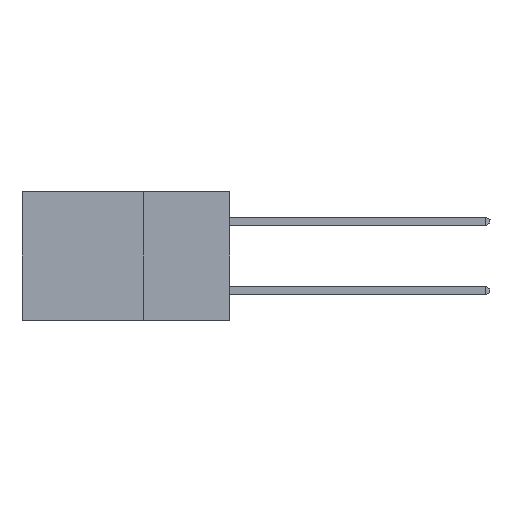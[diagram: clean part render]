
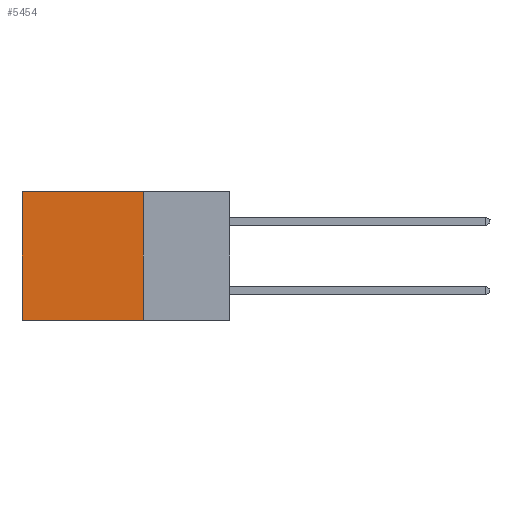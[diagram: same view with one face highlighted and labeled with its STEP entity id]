
A CAD part, left-side view. The second image highlights one B-rep face of the part: STEP entity #5454.
In plain terms, the highlighted planar face has unit normal (-1, 0, 0).
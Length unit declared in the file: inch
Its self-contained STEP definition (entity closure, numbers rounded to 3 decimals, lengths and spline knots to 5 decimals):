
#458 = CARTESIAN_POINT ( 'NONE',  ( 0.298, 0.25, 0. ) ) ;
#592 = PLANE ( 'NONE',  #22406 ) ;
#1752 = EDGE_CURVE ( 'NONE', #11318, #9129, #14719, .T. ) ;
#2717 = CARTESIAN_POINT ( 'NONE',  ( 0.298, 0.25, -0.37 ) ) ;
#3221 = CARTESIAN_POINT ( 'NONE',  ( 0.298, 0.6, -0.37 ) ) ;
#4415 = CARTESIAN_POINT ( 'NONE',  ( 0.298, 0.25, 0. ) ) ;
#4504 = EDGE_CURVE ( 'NONE', #11514, #21722, #30397, .T. ) ;
#4523 = DIRECTION ( 'NONE',  ( 0., 1., 0. ) ) ;
#5454 = ADVANCED_FACE ( 'NONE', ( #21950 ), #592, .F. ) ;
#5462 = LINE ( 'NONE', #11968, #6195 ) ;
#6195 = VECTOR ( 'NONE', #26225, 39.37008 ) ;
#7953 = CARTESIAN_POINT ( 'NONE',  ( 0.298, 0.6, 0. ) ) ;
#9041 = DIRECTION ( 'NONE',  ( 0., 0., -1. ) ) ;
#9129 = VERTEX_POINT ( 'NONE', #3221 ) ;
#10931 = VECTOR ( 'NONE', #4523, 39.37008 ) ;
#11121 = ORIENTED_EDGE ( 'NONE', *, *, #1752, .T. ) ;
#11318 = VERTEX_POINT ( 'NONE', #7953 ) ;
#11514 = VERTEX_POINT ( 'NONE', #4415 ) ;
#11968 = CARTESIAN_POINT ( 'NONE',  ( 0.298, 0.25, 0. ) ) ;
#13831 = VECTOR ( 'NONE', #21109, 39.37008 ) ;
#14478 = ORIENTED_EDGE ( 'NONE', *, *, #18356, .T. ) ;
#14674 = DIRECTION ( 'NONE',  ( 1., 0., 0. ) ) ;
#14719 = LINE ( 'NONE', #24206, #28016 ) ;
#15140 = EDGE_CURVE ( 'NONE', #21722, #9129, #16534, .T. ) ;
#16534 = LINE ( 'NONE', #18794, #10931 ) ;
#16572 = EDGE_LOOP ( 'NONE', ( #11121, #18132, #18493, #14478 ) ) ;
#18132 = ORIENTED_EDGE ( 'NONE', *, *, #15140, .F. ) ;
#18356 = EDGE_CURVE ( 'NONE', #11514, #11318, #5462, .T. ) ;
#18493 = ORIENTED_EDGE ( 'NONE', *, *, #4504, .F. ) ;
#18794 = CARTESIAN_POINT ( 'NONE',  ( 0.298, 0.25, -0.37 ) ) ;
#21109 = DIRECTION ( 'NONE',  ( 0., 0., -1. ) ) ;
#21709 = DIRECTION ( 'NONE',  ( 0., 0., -1. ) ) ;
#21722 = VERTEX_POINT ( 'NONE', #2717 ) ;
#21950 = FACE_OUTER_BOUND ( 'NONE', #16572, .T. ) ;
#22406 = AXIS2_PLACEMENT_3D ( 'NONE', #25410, #14674, #21709 ) ;
#24206 = CARTESIAN_POINT ( 'NONE',  ( 0.298, 0.6, 0. ) ) ;
#25410 = CARTESIAN_POINT ( 'NONE',  ( 0.298, 0.25, 0. ) ) ;
#26225 = DIRECTION ( 'NONE',  ( 0., 1., 0. ) ) ;
#28016 = VECTOR ( 'NONE', #9041, 39.37008 ) ;
#30397 = LINE ( 'NONE', #458, #13831 ) ;
